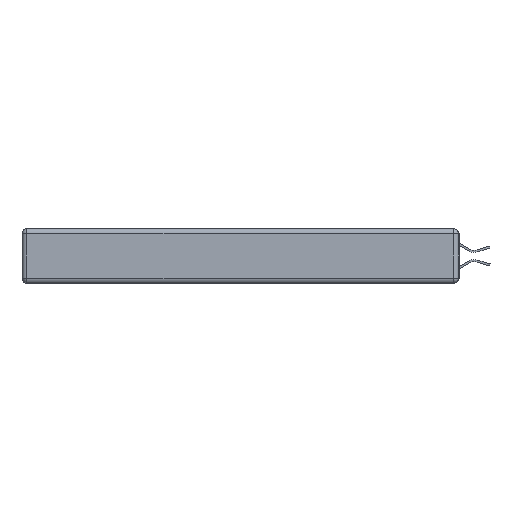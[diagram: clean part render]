
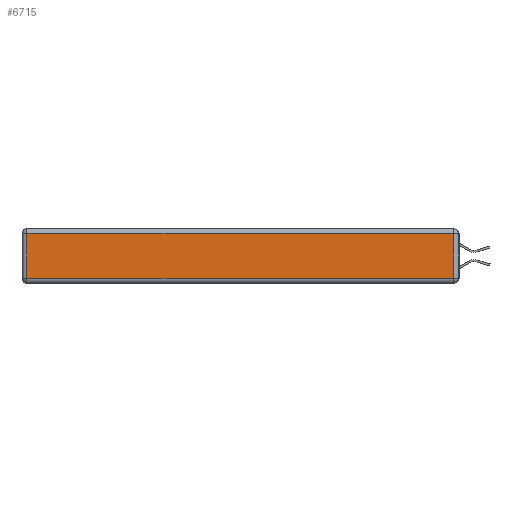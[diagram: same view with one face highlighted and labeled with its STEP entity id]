
A CAD part, left-side view. The second image highlights one B-rep face of the part: STEP entity #6715.
In plain terms, the highlighted planar face has unit normal (-1, 0, 0).
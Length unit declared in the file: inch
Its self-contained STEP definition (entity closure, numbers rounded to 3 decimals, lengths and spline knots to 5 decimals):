
#213 = DIRECTION ( 'NONE',  ( 0., -1., 0. ) ) ;
#456 = VERTEX_POINT ( 'NONE', #15721 ) ;
#461 = CARTESIAN_POINT ( 'NONE',  ( 0., 2.72, -0.313 ) ) ;
#516 = ORIENTED_EDGE ( 'NONE', *, *, #738, .T. ) ;
#623 = LINE ( 'NONE', #1794, #5046 ) ;
#738 = EDGE_CURVE ( 'NONE', #6942, #16464, #10436, .T. ) ;
#1794 = CARTESIAN_POINT ( 'NONE',  ( 0., 2.75, -0.03 ) ) ;
#1921 = VECTOR ( 'NONE', #213, 39.37008 ) ;
#2023 = VECTOR ( 'NONE', #6597, 39.37008 ) ;
#2359 = EDGE_CURVE ( 'NONE', #456, #6918, #11082, .T. ) ;
#3312 = ORIENTED_EDGE ( 'NONE', *, *, #6966, .T. ) ;
#4445 = DIRECTION ( 'NONE',  ( 0., 0., 1. ) ) ;
#4798 = PLANE ( 'NONE',  #10136 ) ;
#5046 = VECTOR ( 'NONE', #11970, 39.37008 ) ;
#5373 = CARTESIAN_POINT ( 'NONE',  ( 0., 0.03, -0.03 ) ) ;
#6597 = DIRECTION ( 'NONE',  ( 0., 0., 1. ) ) ;
#6683 = CARTESIAN_POINT ( 'NONE',  ( 0., 0.03, -0.343 ) ) ;
#6715 = ADVANCED_FACE ( 'NONE', ( #7213 ), #4798, .T. ) ;
#6918 = VERTEX_POINT ( 'NONE', #461 ) ;
#6942 = VERTEX_POINT ( 'NONE', #11646 ) ;
#6966 = EDGE_CURVE ( 'NONE', #6918, #6942, #10628, .T. ) ;
#7213 = FACE_OUTER_BOUND ( 'NONE', #10574, .T. ) ;
#8395 = DIRECTION ( 'NONE',  ( -1., 0., 0. ) ) ;
#10136 = AXIS2_PLACEMENT_3D ( 'NONE', #14996, #8395, #4445 ) ;
#10436 = LINE ( 'NONE', #6683, #2023 ) ;
#10574 = EDGE_LOOP ( 'NONE', ( #3312, #516, #12854, #12625 ) ) ;
#10628 = LINE ( 'NONE', #13131, #1921 ) ;
#11082 = LINE ( 'NONE', #13757, #13295 ) ;
#11646 = CARTESIAN_POINT ( 'NONE',  ( 0., 0.03, -0.313 ) ) ;
#11970 = DIRECTION ( 'NONE',  ( 0., 1., 0. ) ) ;
#12625 = ORIENTED_EDGE ( 'NONE', *, *, #2359, .T. ) ;
#12854 = ORIENTED_EDGE ( 'NONE', *, *, #15445, .T. ) ;
#13131 = CARTESIAN_POINT ( 'NONE',  ( 0., 0., -0.313 ) ) ;
#13295 = VECTOR ( 'NONE', #15100, 39.37008 ) ;
#13757 = CARTESIAN_POINT ( 'NONE',  ( 0., 2.72, -0.343 ) ) ;
#14996 = CARTESIAN_POINT ( 'NONE',  ( 0., 0., -0.343 ) ) ;
#15100 = DIRECTION ( 'NONE',  ( 0., 0., -1. ) ) ;
#15445 = EDGE_CURVE ( 'NONE', #16464, #456, #623, .T. ) ;
#15721 = CARTESIAN_POINT ( 'NONE',  ( 0., 2.72, -0.03 ) ) ;
#16464 = VERTEX_POINT ( 'NONE', #5373 ) ;
